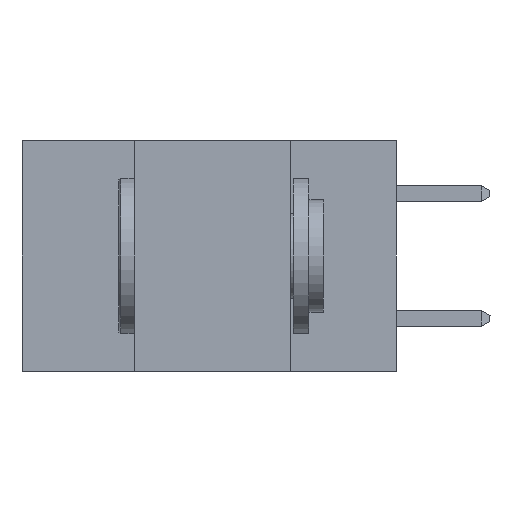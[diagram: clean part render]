
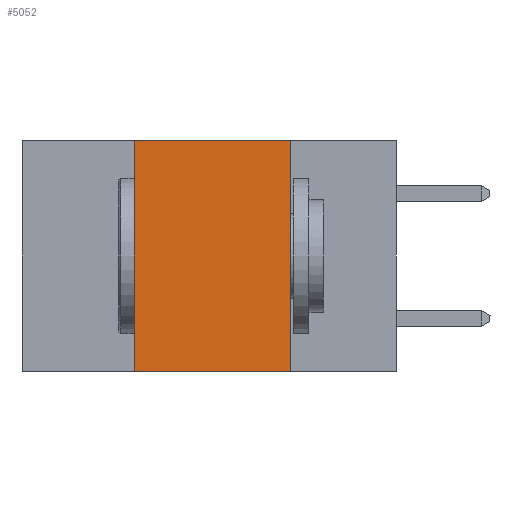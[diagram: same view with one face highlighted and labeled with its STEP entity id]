
A CAD part, left-side view. The second image highlights one B-rep face of the part: STEP entity #5052.
In plain terms, the highlighted planar face has unit normal (-1, 0, 0).
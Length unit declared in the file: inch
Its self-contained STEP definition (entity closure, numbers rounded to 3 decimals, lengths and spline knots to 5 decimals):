
#412 = CARTESIAN_POINT ( 'NONE',  ( 0., 0.42, -0.37 ) ) ;
#745 = VECTOR ( 'NONE', #9514, 39.37008 ) ;
#797 = VERTEX_POINT ( 'NONE', #7375 ) ;
#1078 = EDGE_CURVE ( 'NONE', #797, #5652, #8590, .T. ) ;
#1359 = LINE ( 'NONE', #4591, #5911 ) ;
#1954 = VERTEX_POINT ( 'NONE', #412 ) ;
#2902 = CARTESIAN_POINT ( 'NONE',  ( 0., 0.6, 0. ) ) ;
#3241 = CARTESIAN_POINT ( 'NONE',  ( 0., 0.17, -0.37 ) ) ;
#3527 = VECTOR ( 'NONE', #9701, 39.37008 ) ;
#3656 = CARTESIAN_POINT ( 'NONE',  ( 0., 0.17, -0.37 ) ) ;
#3808 = DIRECTION ( 'NONE',  ( 0., 0., -1. ) ) ;
#4591 = CARTESIAN_POINT ( 'NONE',  ( 0., 0.42, -0.37 ) ) ;
#5052 = ADVANCED_FACE ( 'NONE', ( #10835 ), #7336, .F. ) ;
#5185 = CARTESIAN_POINT ( 'NONE',  ( 0., 0.6, 0. ) ) ;
#5386 = CARTESIAN_POINT ( 'NONE',  ( 0., 0.6, -0.37 ) ) ;
#5477 = DIRECTION ( 'NONE',  ( 0., 0., 1. ) ) ;
#5652 = VERTEX_POINT ( 'NONE', #3656 ) ;
#5911 = VECTOR ( 'NONE', #5477, 39.37008 ) ;
#5959 = CARTESIAN_POINT ( 'NONE',  ( 0., 0.42, 0. ) ) ;
#6267 = VECTOR ( 'NONE', #10148, 39.37008 ) ;
#7336 = PLANE ( 'NONE',  #10679 ) ;
#7375 = CARTESIAN_POINT ( 'NONE',  ( 0., 0.17, 0. ) ) ;
#7676 = LINE ( 'NONE', #5185, #745 ) ;
#7715 = ORIENTED_EDGE ( 'NONE', *, *, #10149, .F. ) ;
#8008 = ORIENTED_EDGE ( 'NONE', *, *, #11254, .F. ) ;
#8499 = LINE ( 'NONE', #5386, #3527 ) ;
#8544 = ORIENTED_EDGE ( 'NONE', *, *, #1078, .F. ) ;
#8590 = LINE ( 'NONE', #3241, #6267 ) ;
#9079 = DIRECTION ( 'NONE',  ( 1., 0., 0. ) ) ;
#9350 = EDGE_LOOP ( 'NONE', ( #8544, #8008, #7715, #10873 ) ) ;
#9514 = DIRECTION ( 'NONE',  ( 0., -1., 0. ) ) ;
#9701 = DIRECTION ( 'NONE',  ( 0., -1., 0. ) ) ;
#10148 = DIRECTION ( 'NONE',  ( 0., 0., -1. ) ) ;
#10149 = EDGE_CURVE ( 'NONE', #1954, #11167, #1359, .T. ) ;
#10679 = AXIS2_PLACEMENT_3D ( 'NONE', #2902, #9079, #3808 ) ;
#10706 = EDGE_CURVE ( 'NONE', #1954, #5652, #8499, .T. ) ;
#10835 = FACE_OUTER_BOUND ( 'NONE', #9350, .T. ) ;
#10873 = ORIENTED_EDGE ( 'NONE', *, *, #10706, .T. ) ;
#11167 = VERTEX_POINT ( 'NONE', #5959 ) ;
#11254 = EDGE_CURVE ( 'NONE', #11167, #797, #7676, .T. ) ;
